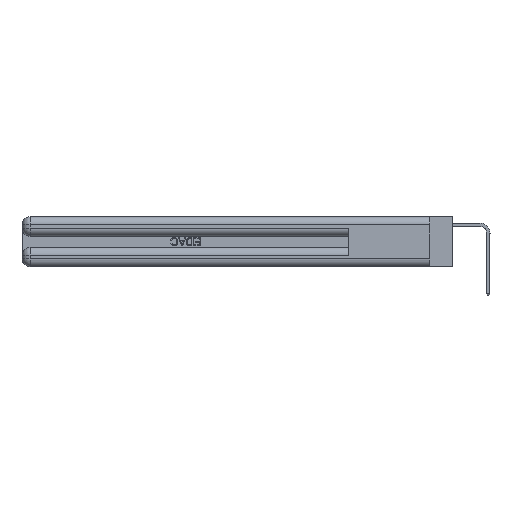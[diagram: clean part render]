
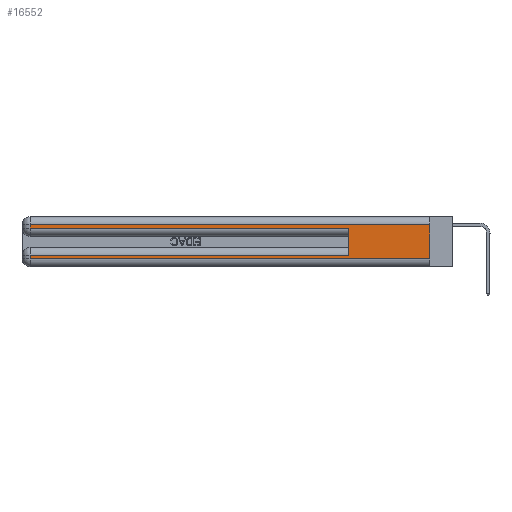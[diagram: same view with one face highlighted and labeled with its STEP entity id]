
A CAD part, left-side view. The second image highlights one B-rep face of the part: STEP entity #16552.
In plain terms, the highlighted planar face has unit normal (-1, 0, 0).
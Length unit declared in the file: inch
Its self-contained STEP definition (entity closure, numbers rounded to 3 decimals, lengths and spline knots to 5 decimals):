
#340 = VECTOR ( 'NONE', #3043, 39.37008 ) ;
#792 = CARTESIAN_POINT ( 'NONE',  ( 0., 2.94, 0.085 ) ) ;
#900 = DIRECTION ( 'NONE',  ( 0., 0., -1. ) ) ;
#1352 = DIRECTION ( 'NONE',  ( 0., 1., 0. ) ) ;
#1411 = VECTOR ( 'NONE', #1352, 39.37008 ) ;
#1447 = DIRECTION ( 'NONE',  ( 0., 0., -1. ) ) ;
#2067 = VERTEX_POINT ( 'NONE', #3013 ) ;
#2625 = CARTESIAN_POINT ( 'NONE',  ( 0., 0.6, 0.285 ) ) ;
#3013 = CARTESIAN_POINT ( 'NONE',  ( 0., 0., 0.31 ) ) ;
#3043 = DIRECTION ( 'NONE',  ( 0., 0., 1. ) ) ;
#3279 = LINE ( 'NONE', #17270, #32379 ) ;
#3974 = CARTESIAN_POINT ( 'NONE',  ( 0., 0., 0.06 ) ) ;
#4791 = ORIENTED_EDGE ( 'NONE', *, *, #17302, .T. ) ;
#5199 = CARTESIAN_POINT ( 'NONE',  ( 0., 0.6, 0.085 ) ) ;
#6548 = ORIENTED_EDGE ( 'NONE', *, *, #30495, .T. ) ;
#6815 = VERTEX_POINT ( 'NONE', #792 ) ;
#7596 = ORIENTED_EDGE ( 'NONE', *, *, #27200, .F. ) ;
#9375 = ORIENTED_EDGE ( 'NONE', *, *, #12935, .T. ) ;
#10856 = EDGE_CURVE ( 'NONE', #30910, #23705, #24962, .T. ) ;
#11670 = CARTESIAN_POINT ( 'NONE',  ( 0., 0., 0.37 ) ) ;
#11897 = LINE ( 'NONE', #14583, #18153 ) ;
#11999 = DIRECTION ( 'NONE',  ( 0., -1., 0. ) ) ;
#12223 = LINE ( 'NONE', #17304, #1411 ) ;
#12365 = FACE_OUTER_BOUND ( 'NONE', #20733, .T. ) ;
#12522 = ORIENTED_EDGE ( 'NONE', *, *, #34072, .T. ) ;
#12935 = EDGE_CURVE ( 'NONE', #15933, #33693, #34152, .T. ) ;
#13019 = VECTOR ( 'NONE', #17839, 39.37008 ) ;
#13380 = ORIENTED_EDGE ( 'NONE', *, *, #13990, .F. ) ;
#13990 = EDGE_CURVE ( 'NONE', #2067, #23705, #24180, .T. ) ;
#14152 = AXIS2_PLACEMENT_3D ( 'NONE', #11670, #30248, #14391 ) ;
#14391 = DIRECTION ( 'NONE',  ( 0., 0., -1. ) ) ;
#14583 = CARTESIAN_POINT ( 'NONE',  ( 0., 2.94, 0.37 ) ) ;
#14604 = ORIENTED_EDGE ( 'NONE', *, *, #18393, .T. ) ;
#15181 = VERTEX_POINT ( 'NONE', #32646 ) ;
#15933 = VERTEX_POINT ( 'NONE', #27840 ) ;
#16552 = ADVANCED_FACE ( 'NONE', ( #12365 ), #24889, .F. ) ;
#17159 = VECTOR ( 'NONE', #900, 39.37008 ) ;
#17175 = CARTESIAN_POINT ( 'NONE',  ( 0., 2.94, 0.37 ) ) ;
#17270 = CARTESIAN_POINT ( 'NONE',  ( 0., 0., 0.085 ) ) ;
#17302 = EDGE_CURVE ( 'NONE', #6815, #30910, #11897, .T. ) ;
#17304 = CARTESIAN_POINT ( 'NONE',  ( 0., 0., 0.31 ) ) ;
#17839 = DIRECTION ( 'NONE',  ( 0., -1., 0. ) ) ;
#18153 = VECTOR ( 'NONE', #27760, 39.37008 ) ;
#18393 = EDGE_CURVE ( 'NONE', #23362, #6815, #3279, .T. ) ;
#19551 = VECTOR ( 'NONE', #1447, 39.37008 ) ;
#20058 = CARTESIAN_POINT ( 'NONE',  ( 0., 0., 0.06 ) ) ;
#20733 = EDGE_LOOP ( 'NONE', ( #13380, #6548, #12522, #9375, #7596, #14604, #4791, #33585 ) ) ;
#21652 = CARTESIAN_POINT ( 'NONE',  ( 0., 0.6, 0.145 ) ) ;
#23362 = VERTEX_POINT ( 'NONE', #5199 ) ;
#23705 = VERTEX_POINT ( 'NONE', #20058 ) ;
#24132 = VECTOR ( 'NONE', #11999, 39.37008 ) ;
#24180 = LINE ( 'NONE', #32720, #17159 ) ;
#24889 = PLANE ( 'NONE',  #14152 ) ;
#24962 = LINE ( 'NONE', #3974, #24132 ) ;
#26778 = CARTESIAN_POINT ( 'NONE',  ( 0., 2.94, 0.06 ) ) ;
#27200 = EDGE_CURVE ( 'NONE', #23362, #33693, #28600, .T. ) ;
#27760 = DIRECTION ( 'NONE',  ( 0., 0., -1. ) ) ;
#27808 = DIRECTION ( 'NONE',  ( 0., 1., 0. ) ) ;
#27840 = CARTESIAN_POINT ( 'NONE',  ( 0., 2.94, 0.285 ) ) ;
#28600 = LINE ( 'NONE', #21652, #340 ) ;
#30248 = DIRECTION ( 'NONE',  ( 1., 0., 0. ) ) ;
#30495 = EDGE_CURVE ( 'NONE', #2067, #15181, #12223, .T. ) ;
#30910 = VERTEX_POINT ( 'NONE', #26778 ) ;
#31030 = CARTESIAN_POINT ( 'NONE',  ( 0., 0., 0.285 ) ) ;
#32379 = VECTOR ( 'NONE', #27808, 39.37008 ) ;
#32646 = CARTESIAN_POINT ( 'NONE',  ( 0., 2.94, 0.31 ) ) ;
#32720 = CARTESIAN_POINT ( 'NONE',  ( 0., 0., 0.37 ) ) ;
#33585 = ORIENTED_EDGE ( 'NONE', *, *, #10856, .T. ) ;
#33645 = LINE ( 'NONE', #17175, #19551 ) ;
#33693 = VERTEX_POINT ( 'NONE', #2625 ) ;
#34072 = EDGE_CURVE ( 'NONE', #15181, #15933, #33645, .T. ) ;
#34152 = LINE ( 'NONE', #31030, #13019 ) ;
